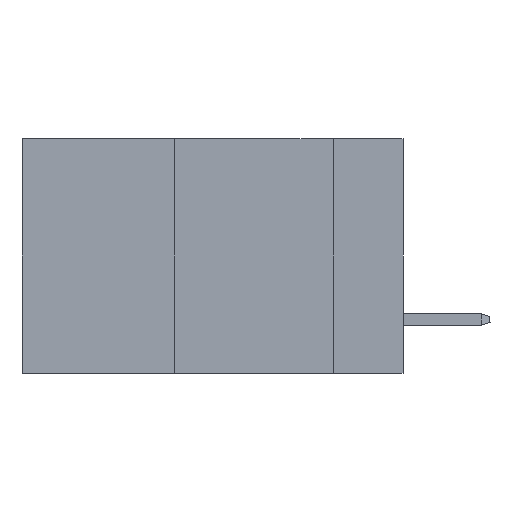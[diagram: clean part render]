
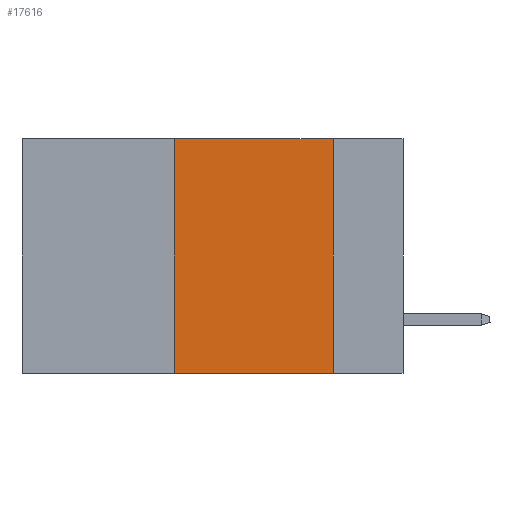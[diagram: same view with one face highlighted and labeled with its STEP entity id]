
A CAD part, left-side view. The second image highlights one B-rep face of the part: STEP entity #17616.
In plain terms, the highlighted planar face has unit normal (-1, 0, 0).
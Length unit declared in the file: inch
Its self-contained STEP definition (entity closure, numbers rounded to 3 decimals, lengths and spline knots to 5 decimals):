
#207 = VECTOR ( 'NONE', #11710, 39.37008 ) ;
#512 = ORIENTED_EDGE ( 'NONE', *, *, #10006, .F. ) ;
#802 = AXIS2_PLACEMENT_3D ( 'NONE', #22160, #18021, #26633 ) ;
#1435 = ORIENTED_EDGE ( 'NONE', *, *, #28650, .F. ) ;
#1569 = DIRECTION ( 'NONE',  ( 0., -1., 0. ) ) ;
#1864 = CARTESIAN_POINT ( 'NONE',  ( 0., 0.6, 0. ) ) ;
#3719 = LINE ( 'NONE', #10701, #26800 ) ;
#4020 = VECTOR ( 'NONE', #11611, 39.37008 ) ;
#4221 = PLANE ( 'NONE',  #802 ) ;
#7118 = CARTESIAN_POINT ( 'NONE',  ( 0., 0.36, -0.37 ) ) ;
#7851 = CARTESIAN_POINT ( 'NONE',  ( 0., 0.36, 0. ) ) ;
#8490 = FACE_OUTER_BOUND ( 'NONE', #14372, .T. ) ;
#9079 = CARTESIAN_POINT ( 'NONE',  ( 0., 0.6, -0.37 ) ) ;
#9449 = LINE ( 'NONE', #20553, #207 ) ;
#9710 = VERTEX_POINT ( 'NONE', #10865 ) ;
#9879 = DIRECTION ( 'NONE',  ( 0., 0., -1. ) ) ;
#9962 = EDGE_CURVE ( 'NONE', #15528, #9710, #29155, .T. ) ;
#10006 = EDGE_CURVE ( 'NONE', #20140, #15528, #9449, .T. ) ;
#10701 = CARTESIAN_POINT ( 'NONE',  ( 0., 0.11, 0. ) ) ;
#10865 = CARTESIAN_POINT ( 'NONE',  ( 0., 0.11, 0. ) ) ;
#11611 = DIRECTION ( 'NONE',  ( 0., -1., 0. ) ) ;
#11710 = DIRECTION ( 'NONE',  ( 0., 0., 1. ) ) ;
#14372 = EDGE_LOOP ( 'NONE', ( #1435, #29159, #512, #19795 ) ) ;
#15222 = VECTOR ( 'NONE', #1569, 39.37008 ) ;
#15528 = VERTEX_POINT ( 'NONE', #7851 ) ;
#16788 = CARTESIAN_POINT ( 'NONE',  ( 0., 0.11, -0.37 ) ) ;
#17616 = ADVANCED_FACE ( 'NONE', ( #8490 ), #4221, .F. ) ;
#18021 = DIRECTION ( 'NONE',  ( 1., 0., 0. ) ) ;
#19795 = ORIENTED_EDGE ( 'NONE', *, *, #27569, .T. ) ;
#20140 = VERTEX_POINT ( 'NONE', #7118 ) ;
#20553 = CARTESIAN_POINT ( 'NONE',  ( 0., 0.36, 0. ) ) ;
#22160 = CARTESIAN_POINT ( 'NONE',  ( 0., 0.6, 0. ) ) ;
#22825 = VERTEX_POINT ( 'NONE', #16788 ) ;
#26633 = DIRECTION ( 'NONE',  ( 0., 0., -1. ) ) ;
#26800 = VECTOR ( 'NONE', #9879, 39.37008 ) ;
#27569 = EDGE_CURVE ( 'NONE', #20140, #22825, #29803, .T. ) ;
#28650 = EDGE_CURVE ( 'NONE', #9710, #22825, #3719, .T. ) ;
#29155 = LINE ( 'NONE', #1864, #15222 ) ;
#29159 = ORIENTED_EDGE ( 'NONE', *, *, #9962, .F. ) ;
#29803 = LINE ( 'NONE', #9079, #4020 ) ;
